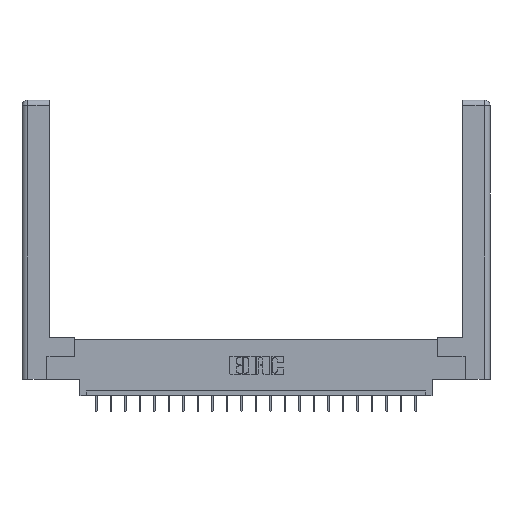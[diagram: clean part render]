
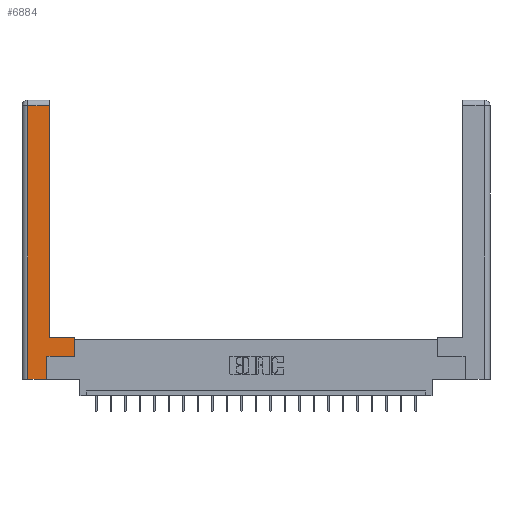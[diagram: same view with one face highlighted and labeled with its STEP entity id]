
A CAD part, top view. The second image highlights one B-rep face of the part: STEP entity #6884.
In plain terms, the highlighted planar face has unit normal (0, 0, 1).
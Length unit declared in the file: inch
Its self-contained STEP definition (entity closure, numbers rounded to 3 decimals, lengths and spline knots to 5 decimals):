
#512 = VECTOR ( 'NONE', #5799, 39.37008 ) ;
#800 = DIRECTION ( 'NONE',  ( -1., 0., 0. ) ) ;
#986 = ORIENTED_EDGE ( 'NONE', *, *, #8460, .T. ) ;
#1429 = VERTEX_POINT ( 'NONE', #9862 ) ;
#1675 = VERTEX_POINT ( 'NONE', #11921 ) ;
#1707 = CARTESIAN_POINT ( 'NONE',  ( 0.265, 0., 0. ) ) ;
#2058 = DIRECTION ( 'NONE',  ( 0., 1., 0. ) ) ;
#2286 = VERTEX_POINT ( 'NONE', #18077 ) ;
#2702 = VECTOR ( 'NONE', #2883, 39.37008 ) ;
#2883 = DIRECTION ( 'NONE',  ( -1., 0., 0. ) ) ;
#2955 = LINE ( 'NONE', #10644, #5942 ) ;
#3298 = CARTESIAN_POINT ( 'NONE',  ( 0.295, 0.45, 0. ) ) ;
#3743 = VERTEX_POINT ( 'NONE', #5511 ) ;
#4285 = ORIENTED_EDGE ( 'NONE', *, *, #4920, .T. ) ;
#4920 = EDGE_CURVE ( 'NONE', #3743, #1675, #14674, .T. ) ;
#4954 = EDGE_CURVE ( 'NONE', #1429, #2286, #9326, .T. ) ;
#5511 = CARTESIAN_POINT ( 'NONE',  ( 0.0615, 2.94, 0. ) ) ;
#5660 = VECTOR ( 'NONE', #2058, 39.37008 ) ;
#5787 = VECTOR ( 'NONE', #13795, 39.37008 ) ;
#5799 = DIRECTION ( 'NONE',  ( 0., 1., 0. ) ) ;
#5942 = VECTOR ( 'NONE', #10468, 39.37008 ) ;
#6203 = ORIENTED_EDGE ( 'NONE', *, *, #14550, .T. ) ;
#6395 = LINE ( 'NONE', #1707, #13969 ) ;
#6884 = ADVANCED_FACE ( 'NONE', ( #18147 ), #21102, .F. ) ;
#7392 = DIRECTION ( 'NONE',  ( 0., 0., -1. ) ) ;
#7602 = VERTEX_POINT ( 'NONE', #20526 ) ;
#7604 = CARTESIAN_POINT ( 'NONE',  ( 0., 0., 0. ) ) ;
#7642 = EDGE_CURVE ( 'NONE', #2286, #8041, #2955, .T. ) ;
#8041 = VERTEX_POINT ( 'NONE', #20122 ) ;
#8333 = LINE ( 'NONE', #21121, #512 ) ;
#8460 = EDGE_CURVE ( 'NONE', #20207, #3743, #22177, .T. ) ;
#9326 = LINE ( 'NONE', #11970, #5787 ) ;
#9862 = CARTESIAN_POINT ( 'NONE',  ( 0.265, 0., 0. ) ) ;
#10176 = ORIENTED_EDGE ( 'NONE', *, *, #17892, .T. ) ;
#10226 = ORIENTED_EDGE ( 'NONE', *, *, #7642, .T. ) ;
#10468 = DIRECTION ( 'NONE',  ( 1., 0., 0. ) ) ;
#10559 = EDGE_CURVE ( 'NONE', #1675, #1429, #6395, .T. ) ;
#10644 = CARTESIAN_POINT ( 'NONE',  ( 0.565, 0.245, 0. ) ) ;
#10852 = VERTEX_POINT ( 'NONE', #3298 ) ;
#11921 = CARTESIAN_POINT ( 'NONE',  ( 0.0615, 0., 0. ) ) ;
#11970 = CARTESIAN_POINT ( 'NONE',  ( 0.265, 0.245, 0. ) ) ;
#13319 = CARTESIAN_POINT ( 'NONE',  ( 0.0615, 0., 0. ) ) ;
#13396 = DIRECTION ( 'NONE',  ( 0., -1., 0. ) ) ;
#13795 = DIRECTION ( 'NONE',  ( 0., 1., 0. ) ) ;
#13969 = VECTOR ( 'NONE', #21061, 39.37008 ) ;
#14082 = EDGE_CURVE ( 'NONE', #8041, #7602, #19717, .T. ) ;
#14550 = EDGE_CURVE ( 'NONE', #10852, #20207, #8333, .T. ) ;
#14674 = LINE ( 'NONE', #13319, #20110 ) ;
#14877 = LINE ( 'NONE', #21991, #20600 ) ;
#15646 = CARTESIAN_POINT ( 'NONE',  ( 0.565, 0.45, 0. ) ) ;
#17175 = ORIENTED_EDGE ( 'NONE', *, *, #10559, .T. ) ;
#17745 = ORIENTED_EDGE ( 'NONE', *, *, #4954, .T. ) ;
#17754 = AXIS2_PLACEMENT_3D ( 'NONE', #7604, #7392, #800 ) ;
#17892 = EDGE_CURVE ( 'NONE', #7602, #10852, #14877, .T. ) ;
#18077 = CARTESIAN_POINT ( 'NONE',  ( 0.265, 0.245, 0. ) ) ;
#18132 = ORIENTED_EDGE ( 'NONE', *, *, #14082, .T. ) ;
#18147 = FACE_OUTER_BOUND ( 'NONE', #20788, .T. ) ;
#18471 = CARTESIAN_POINT ( 'NONE',  ( 0.295, 2.94, 0. ) ) ;
#18529 = CARTESIAN_POINT ( 'NONE',  ( 0.0615, 2.94, 0. ) ) ;
#19717 = LINE ( 'NONE', #15646, #5660 ) ;
#20110 = VECTOR ( 'NONE', #13396, 39.37008 ) ;
#20122 = CARTESIAN_POINT ( 'NONE',  ( 0.565, 0.245, 0. ) ) ;
#20207 = VERTEX_POINT ( 'NONE', #18471 ) ;
#20526 = CARTESIAN_POINT ( 'NONE',  ( 0.565, 0.45, 0. ) ) ;
#20600 = VECTOR ( 'NONE', #22140, 39.37008 ) ;
#20788 = EDGE_LOOP ( 'NONE', ( #6203, #986, #4285, #17175, #17745, #10226, #18132, #10176 ) ) ;
#21061 = DIRECTION ( 'NONE',  ( 1., 0., 0. ) ) ;
#21102 = PLANE ( 'NONE',  #17754 ) ;
#21121 = CARTESIAN_POINT ( 'NONE',  ( 0.295, 3., 0. ) ) ;
#21991 = CARTESIAN_POINT ( 'NONE',  ( 0.295, 0.45, 0. ) ) ;
#22140 = DIRECTION ( 'NONE',  ( -1., 0., 0. ) ) ;
#22177 = LINE ( 'NONE', #18529, #2702 ) ;
